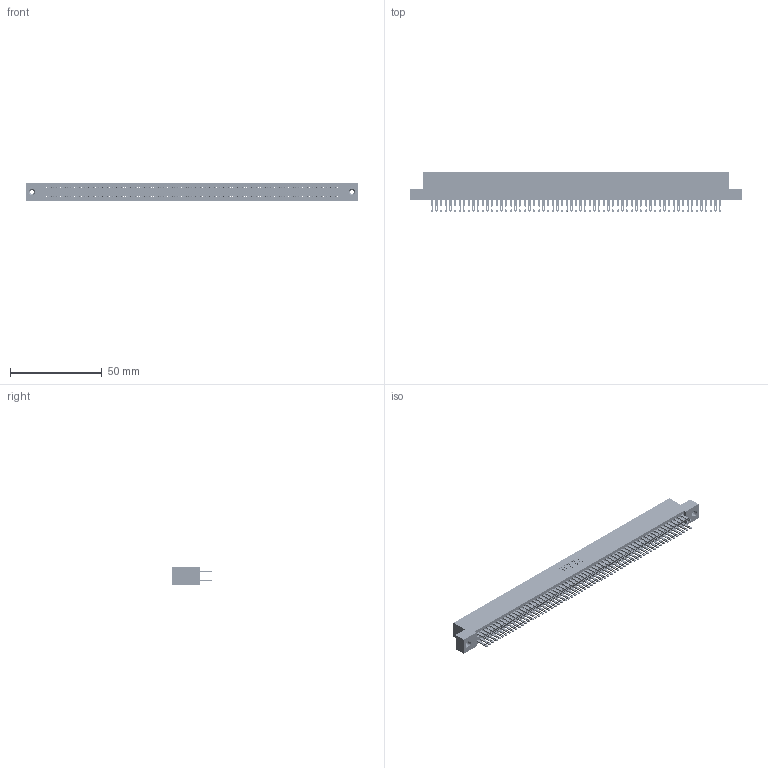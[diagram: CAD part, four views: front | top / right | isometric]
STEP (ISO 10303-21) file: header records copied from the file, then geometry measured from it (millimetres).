
FILE_DESCRIPTION (( 'STEP AP203' ), '1' );
FILE_NAME ('345-126-500-208.STEP', '2018-10-19T12:11:32', ( '' ), ( '' ), 'SwSTEP 2.0', 'SolidWorks 2016', '' );
FILE_SCHEMA (( 'CONFIG_CONTROL_DESIGN' ));
Length unit declared in the file: inch
Products named in the file (4): 345-250-001_345-250-003-102; 345-126-500-208; 345 Part_Flush Mounting Lugs - 0.156 Dia-TI; 345-292-001_345-293-100
Assembly tree (129 placements, depth 2):
  345-126-500-208
    345 Part_Flush Mounting Lugs - 0.156 Dia-TI
    345-292-001_345-293-100  x126
    345-250-001_345-250-003-102  x2
Bounding box: 181.23 x 21.51 x 9.4 mm (x, y, z)
Volume: 18178.2 mm3; surface area: 28575.7 mm2
Topology: 129 solids, 129 shells, 5982 faces, 18243 edges, 12154 vertices
Faces by surface type: plane 3514, cylinder 2452, cone 12, torus 4
Entity records: 47720 total; most frequent: CARTESIAN_POINT 7959, ORIENTED_EDGE 7886, DIRECTION 7021, EDGE_CURVE 3943, LINE 3535, VECTOR 3535, VERTEX_POINT 2624, AXIS2_PLACEMENT_3D 1743
